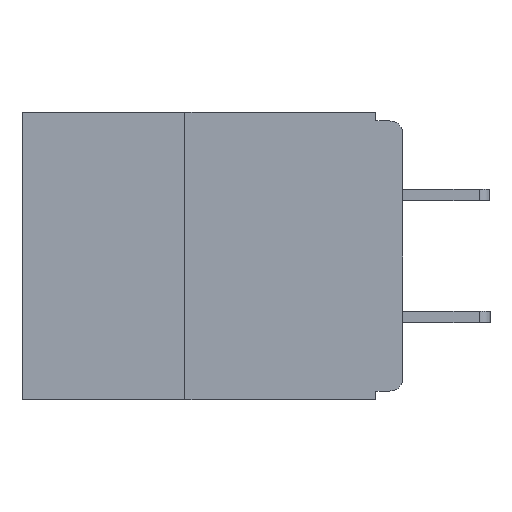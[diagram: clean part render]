
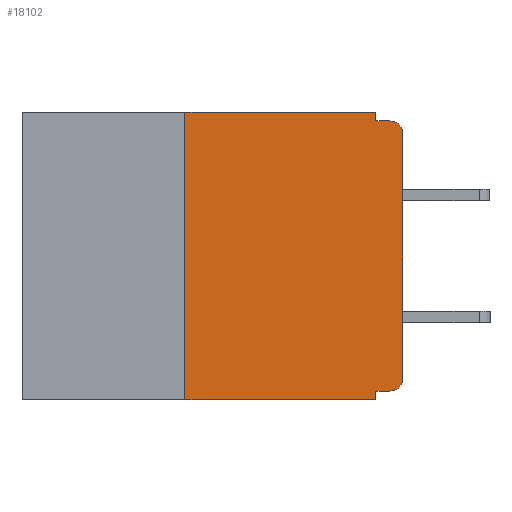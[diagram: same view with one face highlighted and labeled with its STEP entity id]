
A CAD part, left-side view. The second image highlights one B-rep face of the part: STEP entity #18102.
In plain terms, the highlighted planar face has unit normal (-1, 0, 0).
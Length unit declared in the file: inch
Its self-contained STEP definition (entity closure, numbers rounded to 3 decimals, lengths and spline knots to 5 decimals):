
#104 = LINE ( 'NONE', #1951, #18792 ) ;
#342 = ORIENTED_EDGE ( 'NONE', *, *, #17439, .T. ) ;
#394 = CARTESIAN_POINT ( 'NONE',  ( 0., 0., -0.025 ) ) ;
#455 = DIRECTION ( 'NONE',  ( 0., 0., 1. ) ) ;
#513 = CARTESIAN_POINT ( 'NONE',  ( 0., 0.25, -0.33 ) ) ;
#1224 = DIRECTION ( 'NONE',  ( 0., 0., 1. ) ) ;
#1951 = CARTESIAN_POINT ( 'NONE',  ( 0., 0.437, 0. ) ) ;
#2269 = CARTESIAN_POINT ( 'NONE',  ( 0., 0., -0.32 ) ) ;
#2544 = LINE ( 'NONE', #10647, #15856 ) ;
#2694 = AXIS2_PLACEMENT_3D ( 'NONE', #23149, #19775, #9127 ) ;
#2906 = ORIENTED_EDGE ( 'NONE', *, *, #11613, .F. ) ;
#3511 = DIRECTION ( 'NONE',  ( -1., 0., 0. ) ) ;
#3597 = DIRECTION ( 'NONE',  ( 0., -1., 0. ) ) ;
#3612 = CARTESIAN_POINT ( 'NONE',  ( 0., 0., -0.01 ) ) ;
#3683 = VERTEX_POINT ( 'NONE', #8740 ) ;
#4293 = VECTOR ( 'NONE', #1224, 39.37008 ) ;
#4729 = CARTESIAN_POINT ( 'NONE',  ( 0., 0.015, -0.32 ) ) ;
#5162 = DIRECTION ( 'NONE',  ( 0., -1., 0. ) ) ;
#5246 = CARTESIAN_POINT ( 'NONE',  ( 0., 0.437, -0.33 ) ) ;
#5486 = EDGE_CURVE ( 'NONE', #18828, #21407, #2544, .T. ) ;
#5544 = VERTEX_POINT ( 'NONE', #10017 ) ;
#5930 = DIRECTION ( 'NONE',  ( 0., 1., 0. ) ) ;
#6108 = EDGE_CURVE ( 'NONE', #3683, #18343, #19967, .T. ) ;
#6716 = EDGE_CURVE ( 'NONE', #18466, #21407, #21589, .T. ) ;
#6899 = ORIENTED_EDGE ( 'NONE', *, *, #5486, .F. ) ;
#7792 = ORIENTED_EDGE ( 'NONE', *, *, #12677, .T. ) ;
#7973 = EDGE_CURVE ( 'NONE', #18466, #22857, #10198, .T. ) ;
#8069 = CARTESIAN_POINT ( 'NONE',  ( 0., 0.015, -0.305 ) ) ;
#8249 = CIRCLE ( 'NONE', #10211, 0.015 ) ;
#8310 = CARTESIAN_POINT ( 'NONE',  ( 0., 0.015, -0.01 ) ) ;
#8371 = ORIENTED_EDGE ( 'NONE', *, *, #9211, .F. ) ;
#8740 = CARTESIAN_POINT ( 'NONE',  ( 0., 0.031, -0.01 ) ) ;
#8907 = VECTOR ( 'NONE', #22831, 39.37008 ) ;
#9127 = DIRECTION ( 'NONE',  ( 0., 0., -1. ) ) ;
#9211 = EDGE_CURVE ( 'NONE', #22857, #11138, #104, .T. ) ;
#9338 = DIRECTION ( 'NONE',  ( 0., -1., 0. ) ) ;
#9914 = DIRECTION ( 'NONE',  ( 0., 0., -1. ) ) ;
#10017 = CARTESIAN_POINT ( 'NONE',  ( 0., 0., -0.305 ) ) ;
#10198 = LINE ( 'NONE', #513, #19085 ) ;
#10211 = AXIS2_PLACEMENT_3D ( 'NONE', #14365, #3511, #16159 ) ;
#10647 = CARTESIAN_POINT ( 'NONE',  ( 0., 0.031, -0.33 ) ) ;
#10703 = LINE ( 'NONE', #2269, #14871 ) ;
#10812 = DIRECTION ( 'NONE',  ( 0., 0., -1. ) ) ;
#10916 = ORIENTED_EDGE ( 'NONE', *, *, #7973, .F. ) ;
#11138 = VERTEX_POINT ( 'NONE', #11380 ) ;
#11380 = CARTESIAN_POINT ( 'NONE',  ( 0., 0.031, 0. ) ) ;
#11429 = EDGE_LOOP ( 'NONE', ( #16503, #342, #20882, #2906, #8371, #10916, #19793, #6899, #16748, #7792 ) ) ;
#11613 = EDGE_CURVE ( 'NONE', #11138, #3683, #18398, .T. ) ;
#12211 = VECTOR ( 'NONE', #3597, 39.37008 ) ;
#12677 = EDGE_CURVE ( 'NONE', #19018, #5544, #23205, .T. ) ;
#13693 = VERTEX_POINT ( 'NONE', #394 ) ;
#14077 = CARTESIAN_POINT ( 'NONE',  ( 0., 0.031, 0. ) ) ;
#14365 = CARTESIAN_POINT ( 'NONE',  ( 0., 0.015, -0.025 ) ) ;
#14871 = VECTOR ( 'NONE', #5930, 39.37008 ) ;
#15019 = CARTESIAN_POINT ( 'NONE',  ( 0., 0.031, -0.32 ) ) ;
#15718 = CARTESIAN_POINT ( 'NONE',  ( 0., 0., 0. ) ) ;
#15740 = CARTESIAN_POINT ( 'NONE',  ( 0., 0.25, -0.33 ) ) ;
#15793 = EDGE_CURVE ( 'NONE', #5544, #13693, #18670, .T. ) ;
#15856 = VECTOR ( 'NONE', #10812, 39.37008 ) ;
#16159 = DIRECTION ( 'NONE',  ( 0., 0., -1. ) ) ;
#16503 = ORIENTED_EDGE ( 'NONE', *, *, #15793, .T. ) ;
#16748 = ORIENTED_EDGE ( 'NONE', *, *, #22120, .F. ) ;
#16922 = VECTOR ( 'NONE', #5162, 39.37008 ) ;
#16997 = CARTESIAN_POINT ( 'NONE',  ( 0., 0.25, 0. ) ) ;
#17439 = EDGE_CURVE ( 'NONE', #13693, #18343, #8249, .T. ) ;
#18004 = PLANE ( 'NONE',  #2694 ) ;
#18102 = ADVANCED_FACE ( 'NONE', ( #21551 ), #18004, .F. ) ;
#18343 = VERTEX_POINT ( 'NONE', #8310 ) ;
#18398 = LINE ( 'NONE', #14077, #8907 ) ;
#18466 = VERTEX_POINT ( 'NONE', #15740 ) ;
#18670 = LINE ( 'NONE', #15718, #4293 ) ;
#18792 = VECTOR ( 'NONE', #9338, 39.37008 ) ;
#18828 = VERTEX_POINT ( 'NONE', #15019 ) ;
#19018 = VERTEX_POINT ( 'NONE', #4729 ) ;
#19085 = VECTOR ( 'NONE', #455, 39.37008 ) ;
#19671 = AXIS2_PLACEMENT_3D ( 'NONE', #8069, #20520, #9914 ) ;
#19775 = DIRECTION ( 'NONE',  ( 1., 0., 0. ) ) ;
#19793 = ORIENTED_EDGE ( 'NONE', *, *, #6716, .T. ) ;
#19967 = LINE ( 'NONE', #3612, #12211 ) ;
#20520 = DIRECTION ( 'NONE',  ( -1., 0., 0. ) ) ;
#20882 = ORIENTED_EDGE ( 'NONE', *, *, #6108, .F. ) ;
#21407 = VERTEX_POINT ( 'NONE', #21670 ) ;
#21551 = FACE_OUTER_BOUND ( 'NONE', #11429, .T. ) ;
#21589 = LINE ( 'NONE', #5246, #16922 ) ;
#21670 = CARTESIAN_POINT ( 'NONE',  ( 0., 0.031, -0.33 ) ) ;
#22120 = EDGE_CURVE ( 'NONE', #19018, #18828, #10703, .T. ) ;
#22831 = DIRECTION ( 'NONE',  ( 0., 0., -1. ) ) ;
#22857 = VERTEX_POINT ( 'NONE', #16997 ) ;
#23149 = CARTESIAN_POINT ( 'NONE',  ( 0., 0.437, 0. ) ) ;
#23205 = CIRCLE ( 'NONE', #19671, 0.015 ) ;
